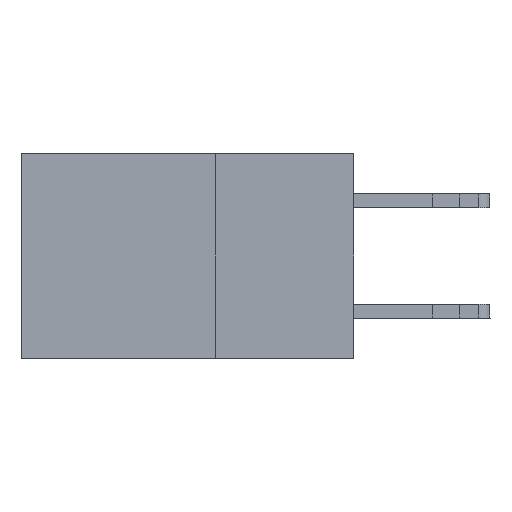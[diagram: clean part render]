
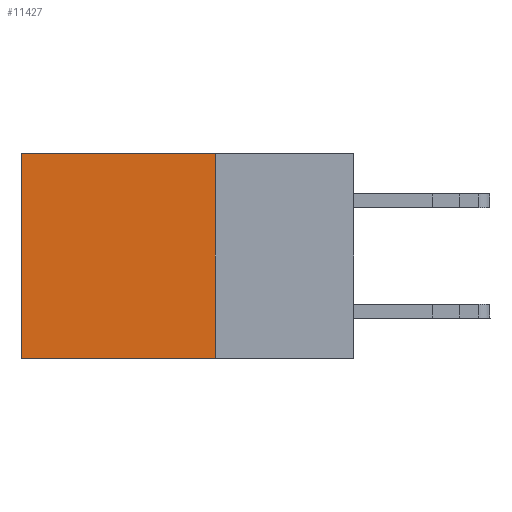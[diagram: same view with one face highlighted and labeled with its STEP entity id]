
A CAD part, left-side view. The second image highlights one B-rep face of the part: STEP entity #11427.
In plain terms, the highlighted planar face has unit normal (-1, 0, 0).
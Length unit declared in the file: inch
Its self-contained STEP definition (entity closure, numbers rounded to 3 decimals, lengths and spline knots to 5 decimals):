
#762 = DIRECTION ( 'NONE',  ( 1., 0., 0. ) ) ;
#1753 = AXIS2_PLACEMENT_3D ( 'NONE', #8816, #762, #16514 ) ;
#1795 = EDGE_CURVE ( 'NONE', #3025, #13435, #3211, .T. ) ;
#2003 = CARTESIAN_POINT ( 'NONE',  ( 0.2875, 0.25, 0. ) ) ;
#2133 = PLANE ( 'NONE',  #1753 ) ;
#2347 = ORIENTED_EDGE ( 'NONE', *, *, #8492, .T. ) ;
#3025 = VERTEX_POINT ( 'NONE', #12168 ) ;
#3138 = CARTESIAN_POINT ( 'NONE',  ( 0.2875, 0.25, 0. ) ) ;
#3211 = LINE ( 'NONE', #4609, #6489 ) ;
#4127 = DIRECTION ( 'NONE',  ( 0., 0., -1. ) ) ;
#4135 = VERTEX_POINT ( 'NONE', #2003 ) ;
#4172 = VERTEX_POINT ( 'NONE', #14832 ) ;
#4358 = DIRECTION ( 'NONE',  ( 0., 1., 0. ) ) ;
#4609 = CARTESIAN_POINT ( 'NONE',  ( 0.2875, 0.25, -0.37 ) ) ;
#5697 = LINE ( 'NONE', #3138, #16382 ) ;
#6489 = VECTOR ( 'NONE', #13813, 39.37008 ) ;
#6634 = LINE ( 'NONE', #7653, #14898 ) ;
#7653 = CARTESIAN_POINT ( 'NONE',  ( 0.2875, 0.6, 0. ) ) ;
#8348 = ORIENTED_EDGE ( 'NONE', *, *, #1795, .F. ) ;
#8492 = EDGE_CURVE ( 'NONE', #4135, #4172, #5697, .T. ) ;
#8816 = CARTESIAN_POINT ( 'NONE',  ( 0.2875, 0.25, 0. ) ) ;
#8946 = EDGE_CURVE ( 'NONE', #4135, #3025, #15638, .T. ) ;
#10020 = ORIENTED_EDGE ( 'NONE', *, *, #15306, .T. ) ;
#10332 = DIRECTION ( 'NONE',  ( 0., 0., -1. ) ) ;
#10353 = ORIENTED_EDGE ( 'NONE', *, *, #8946, .F. ) ;
#11427 = ADVANCED_FACE ( 'NONE', ( #16602 ), #2133, .F. ) ;
#12168 = CARTESIAN_POINT ( 'NONE',  ( 0.2875, 0.25, -0.37 ) ) ;
#12906 = CARTESIAN_POINT ( 'NONE',  ( 0.2875, 0.6, -0.37 ) ) ;
#13001 = CARTESIAN_POINT ( 'NONE',  ( 0.2875, 0.25, 0. ) ) ;
#13435 = VERTEX_POINT ( 'NONE', #12906 ) ;
#13813 = DIRECTION ( 'NONE',  ( 0., 1., 0. ) ) ;
#14832 = CARTESIAN_POINT ( 'NONE',  ( 0.2875, 0.6, 0. ) ) ;
#14898 = VECTOR ( 'NONE', #10332, 39.37008 ) ;
#15306 = EDGE_CURVE ( 'NONE', #4172, #13435, #6634, .T. ) ;
#15638 = LINE ( 'NONE', #13001, #16389 ) ;
#16382 = VECTOR ( 'NONE', #4358, 39.37008 ) ;
#16389 = VECTOR ( 'NONE', #4127, 39.37008 ) ;
#16514 = DIRECTION ( 'NONE',  ( 0., 0., -1. ) ) ;
#16602 = FACE_OUTER_BOUND ( 'NONE', #16787, .T. ) ;
#16787 = EDGE_LOOP ( 'NONE', ( #10020, #8348, #10353, #2347 ) ) ;
